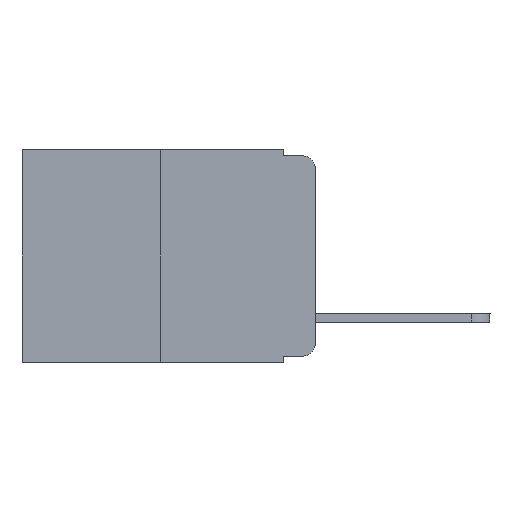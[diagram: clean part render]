
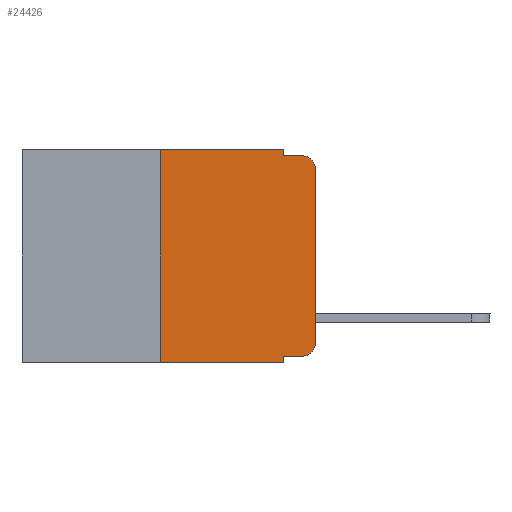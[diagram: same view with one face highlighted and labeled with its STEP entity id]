
A CAD part, left-side view. The second image highlights one B-rep face of the part: STEP entity #24426.
In plain terms, the highlighted planar face has unit normal (-1, 0, 0).
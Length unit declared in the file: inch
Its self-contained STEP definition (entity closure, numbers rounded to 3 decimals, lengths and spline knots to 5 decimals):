
#634 = EDGE_CURVE ( 'NONE', #9906, #17382, #2166, .T. ) ;
#1224 = VECTOR ( 'NONE', #4465, 39.37008 ) ;
#1305 = EDGE_CURVE ( 'NONE', #3431, #7927, #11042, .T. ) ;
#1445 = VERTEX_POINT ( 'NONE', #2435 ) ;
#1550 = EDGE_LOOP ( 'NONE', ( #21756, #10357, #20678, #21571, #21635, #7228, #17734, #18864, #18453, #17184 ) ) ;
#1558 = CARTESIAN_POINT ( 'NONE',  ( 0., 0.473, 0. ) ) ;
#2048 = DIRECTION ( 'NONE',  ( 0., -1., 0. ) ) ;
#2166 = LINE ( 'NONE', #3907, #13100 ) ;
#2340 = LINE ( 'NONE', #3972, #23734 ) ;
#2435 = CARTESIAN_POINT ( 'NONE',  ( 0., 0., -0.313 ) ) ;
#3405 = DIRECTION ( 'NONE',  ( 1., 0., 0. ) ) ;
#3431 = VERTEX_POINT ( 'NONE', #16980 ) ;
#3598 = EDGE_CURVE ( 'NONE', #8968, #17382, #23439, .T. ) ;
#3907 = CARTESIAN_POINT ( 'NONE',  ( 0., 0.473, -0.343 ) ) ;
#3972 = CARTESIAN_POINT ( 'NONE',  ( 0., 0.051, -0.01 ) ) ;
#4465 = DIRECTION ( 'NONE',  ( 0., 0., 1. ) ) ;
#5193 = DIRECTION ( 'NONE',  ( 0., 0., 1. ) ) ;
#5564 = CARTESIAN_POINT ( 'NONE',  ( 0., 0.02, -0.03 ) ) ;
#5654 = PLANE ( 'NONE',  #21404 ) ;
#5885 = CARTESIAN_POINT ( 'NONE',  ( 0., 0.051, -0.01 ) ) ;
#5937 = DIRECTION ( 'NONE',  ( -1., 0., 0. ) ) ;
#6011 = EDGE_CURVE ( 'NONE', #1445, #15812, #13959, .T. ) ;
#6072 = CARTESIAN_POINT ( 'NONE',  ( 0., 0.02, -0.333 ) ) ;
#6277 = EDGE_CURVE ( 'NONE', #9906, #3431, #16562, .T. ) ;
#6349 = DIRECTION ( 'NONE',  ( 0., 0., -1. ) ) ;
#6575 = VERTEX_POINT ( 'NONE', #10912 ) ;
#7078 = EDGE_CURVE ( 'NONE', #7927, #23937, #11099, .T. ) ;
#7228 = ORIENTED_EDGE ( 'NONE', *, *, #6277, .F. ) ;
#7646 = EDGE_CURVE ( 'NONE', #23937, #6575, #2340, .T. ) ;
#7927 = VERTEX_POINT ( 'NONE', #16355 ) ;
#8188 = CARTESIAN_POINT ( 'NONE',  ( 0., 0., -0.03 ) ) ;
#8336 = CARTESIAN_POINT ( 'NONE',  ( 0., 0.02, -0.313 ) ) ;
#8968 = VERTEX_POINT ( 'NONE', #21278 ) ;
#9364 = CARTESIAN_POINT ( 'NONE',  ( 0., 0.051, 0. ) ) ;
#9906 = VERTEX_POINT ( 'NONE', #12176 ) ;
#10357 = ORIENTED_EDGE ( 'NONE', *, *, #11469, .T. ) ;
#10912 = CARTESIAN_POINT ( 'NONE',  ( 0., 0.02, -0.01 ) ) ;
#11042 = LINE ( 'NONE', #1558, #11415 ) ;
#11099 = LINE ( 'NONE', #9364, #13388 ) ;
#11187 = AXIS2_PLACEMENT_3D ( 'NONE', #8336, #23552, #12191 ) ;
#11349 = AXIS2_PLACEMENT_3D ( 'NONE', #5564, #5937, #13566 ) ;
#11415 = VECTOR ( 'NONE', #24137, 39.37008 ) ;
#11469 = EDGE_CURVE ( 'NONE', #15812, #6575, #13326, .T. ) ;
#11579 = DIRECTION ( 'NONE',  ( 0., -1., 0. ) ) ;
#12176 = CARTESIAN_POINT ( 'NONE',  ( 0., 0.25, -0.343 ) ) ;
#12191 = DIRECTION ( 'NONE',  ( 0., 0., -1. ) ) ;
#12865 = LINE ( 'NONE', #16734, #15364 ) ;
#13100 = VECTOR ( 'NONE', #2048, 39.37008 ) ;
#13326 = CIRCLE ( 'NONE', #11349, 0.02 ) ;
#13388 = VECTOR ( 'NONE', #16970, 39.37008 ) ;
#13566 = DIRECTION ( 'NONE',  ( 0., 0., -1. ) ) ;
#13959 = LINE ( 'NONE', #23429, #1224 ) ;
#14532 = VERTEX_POINT ( 'NONE', #6072 ) ;
#15155 = VECTOR ( 'NONE', #6349, 39.37008 ) ;
#15364 = VECTOR ( 'NONE', #22598, 39.37008 ) ;
#15812 = VERTEX_POINT ( 'NONE', #8188 ) ;
#16355 = CARTESIAN_POINT ( 'NONE',  ( 0., 0.051, 0. ) ) ;
#16562 = LINE ( 'NONE', #22294, #20305 ) ;
#16630 = CARTESIAN_POINT ( 'NONE',  ( 0., 0.473, 0. ) ) ;
#16734 = CARTESIAN_POINT ( 'NONE',  ( 0., 0.051, -0.333 ) ) ;
#16970 = DIRECTION ( 'NONE',  ( 0., 0., -1. ) ) ;
#16980 = CARTESIAN_POINT ( 'NONE',  ( 0., 0.25, 0. ) ) ;
#17184 = ORIENTED_EDGE ( 'NONE', *, *, #19408, .T. ) ;
#17382 = VERTEX_POINT ( 'NONE', #17544 ) ;
#17544 = CARTESIAN_POINT ( 'NONE',  ( 0., 0.051, -0.343 ) ) ;
#17734 = ORIENTED_EDGE ( 'NONE', *, *, #634, .T. ) ;
#18364 = CIRCLE ( 'NONE', #11187, 0.02 ) ;
#18453 = ORIENTED_EDGE ( 'NONE', *, *, #22552, .T. ) ;
#18864 = ORIENTED_EDGE ( 'NONE', *, *, #3598, .F. ) ;
#19408 = EDGE_CURVE ( 'NONE', #14532, #1445, #18364, .T. ) ;
#20305 = VECTOR ( 'NONE', #5193, 39.37008 ) ;
#20678 = ORIENTED_EDGE ( 'NONE', *, *, #7646, .F. ) ;
#21278 = CARTESIAN_POINT ( 'NONE',  ( 0., 0.051, -0.333 ) ) ;
#21404 = AXIS2_PLACEMENT_3D ( 'NONE', #16630, #3405, #22748 ) ;
#21571 = ORIENTED_EDGE ( 'NONE', *, *, #7078, .F. ) ;
#21635 = ORIENTED_EDGE ( 'NONE', *, *, #1305, .F. ) ;
#21756 = ORIENTED_EDGE ( 'NONE', *, *, #6011, .T. ) ;
#22238 = FACE_OUTER_BOUND ( 'NONE', #1550, .T. ) ;
#22294 = CARTESIAN_POINT ( 'NONE',  ( 0., 0.25, 0. ) ) ;
#22552 = EDGE_CURVE ( 'NONE', #8968, #14532, #12865, .T. ) ;
#22598 = DIRECTION ( 'NONE',  ( 0., -1., 0. ) ) ;
#22748 = DIRECTION ( 'NONE',  ( 0., 0., -1. ) ) ;
#23320 = CARTESIAN_POINT ( 'NONE',  ( 0., 0.051, 0. ) ) ;
#23429 = CARTESIAN_POINT ( 'NONE',  ( 0., 0., 0. ) ) ;
#23439 = LINE ( 'NONE', #23320, #15155 ) ;
#23552 = DIRECTION ( 'NONE',  ( -1., 0., 0. ) ) ;
#23734 = VECTOR ( 'NONE', #11579, 39.37008 ) ;
#23937 = VERTEX_POINT ( 'NONE', #5885 ) ;
#24137 = DIRECTION ( 'NONE',  ( 0., -1., 0. ) ) ;
#24426 = ADVANCED_FACE ( 'NONE', ( #22238 ), #5654, .F. ) ;
